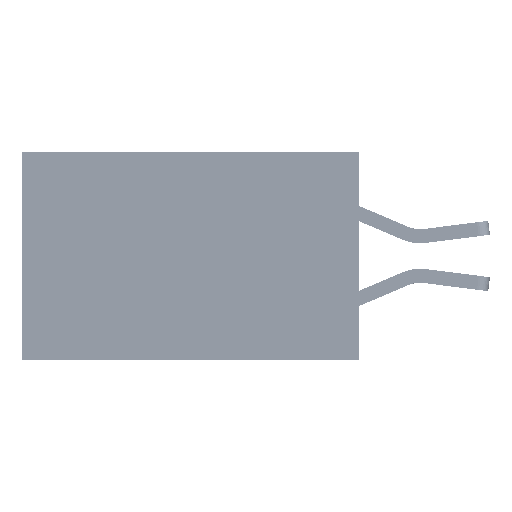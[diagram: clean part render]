
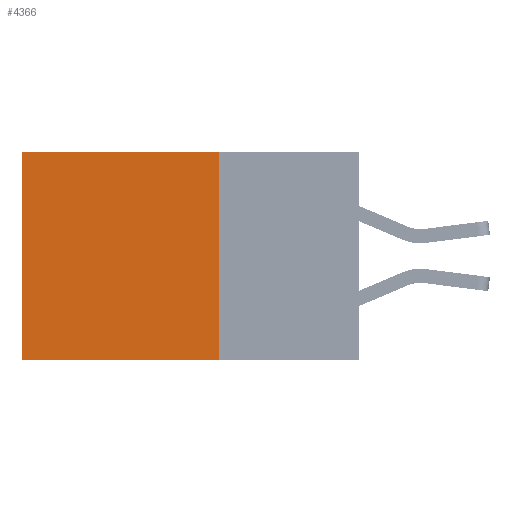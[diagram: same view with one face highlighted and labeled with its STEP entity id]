
A CAD part, left-side view. The second image highlights one B-rep face of the part: STEP entity #4366.
In plain terms, the highlighted planar face has unit normal (-1, 0, 0).
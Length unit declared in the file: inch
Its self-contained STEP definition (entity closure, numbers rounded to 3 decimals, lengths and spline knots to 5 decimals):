
#1500 = DIRECTION ( 'NONE',  ( 1., 0., 0. ) ) ;
#1942 = CARTESIAN_POINT ( 'NONE',  ( 0.2875, 0.25, 0. ) ) ;
#2879 = CARTESIAN_POINT ( 'NONE',  ( 0.2875, 0.6, 0. ) ) ;
#4366 = ADVANCED_FACE ( 'NONE', ( #43454 ), #32549, .F. ) ;
#5172 = CARTESIAN_POINT ( 'NONE',  ( 0.2875, 0.25, 0. ) ) ;
#5240 = EDGE_CURVE ( 'NONE', #18469, #40909, #14969, .T. ) ;
#7207 = CARTESIAN_POINT ( 'NONE',  ( 0.2875, 0.25, -0.37 ) ) ;
#8379 = ORIENTED_EDGE ( 'NONE', *, *, #20305, .T. ) ;
#8395 = VERTEX_POINT ( 'NONE', #41490 ) ;
#9091 = LINE ( 'NONE', #41068, #29549 ) ;
#9686 = DIRECTION ( 'NONE',  ( 0., 1., 0. ) ) ;
#9955 = ORIENTED_EDGE ( 'NONE', *, *, #19773, .F. ) ;
#12868 = CARTESIAN_POINT ( 'NONE',  ( 0.2875, 0.25, 0. ) ) ;
#14969 = LINE ( 'NONE', #12868, #29052 ) ;
#15482 = EDGE_LOOP ( 'NONE', ( #8379, #9955, #20555, #30894 ) ) ;
#15983 = CARTESIAN_POINT ( 'NONE',  ( 0.2875, 0.25, -0.37 ) ) ;
#16377 = EDGE_CURVE ( 'NONE', #18469, #17772, #9091, .T. ) ;
#16797 = DIRECTION ( 'NONE',  ( 0., 0., -1. ) ) ;
#17350 = DIRECTION ( 'NONE',  ( 0., 0., -1. ) ) ;
#17772 = VERTEX_POINT ( 'NONE', #15983 ) ;
#18469 = VERTEX_POINT ( 'NONE', #5172 ) ;
#19448 = DIRECTION ( 'NONE',  ( 0., 1., 0. ) ) ;
#19773 = EDGE_CURVE ( 'NONE', #17772, #8395, #27817, .T. ) ;
#20294 = VECTOR ( 'NONE', #9686, 39.37008 ) ;
#20305 = EDGE_CURVE ( 'NONE', #40909, #8395, #23465, .T. ) ;
#20555 = ORIENTED_EDGE ( 'NONE', *, *, #16377, .F. ) ;
#22098 = DIRECTION ( 'NONE',  ( 0., 0., -1. ) ) ;
#22258 = VECTOR ( 'NONE', #17350, 39.37008 ) ;
#23465 = LINE ( 'NONE', #2879, #22258 ) ;
#27817 = LINE ( 'NONE', #7207, #20294 ) ;
#28334 = AXIS2_PLACEMENT_3D ( 'NONE', #1942, #1500, #22098 ) ;
#29052 = VECTOR ( 'NONE', #19448, 39.37008 ) ;
#29549 = VECTOR ( 'NONE', #16797, 39.37008 ) ;
#30724 = CARTESIAN_POINT ( 'NONE',  ( 0.2875, 0.6, 0. ) ) ;
#30894 = ORIENTED_EDGE ( 'NONE', *, *, #5240, .T. ) ;
#32549 = PLANE ( 'NONE',  #28334 ) ;
#40909 = VERTEX_POINT ( 'NONE', #30724 ) ;
#41068 = CARTESIAN_POINT ( 'NONE',  ( 0.2875, 0.25, 0. ) ) ;
#41490 = CARTESIAN_POINT ( 'NONE',  ( 0.2875, 0.6, -0.37 ) ) ;
#43454 = FACE_OUTER_BOUND ( 'NONE', #15482, .T. ) ;
